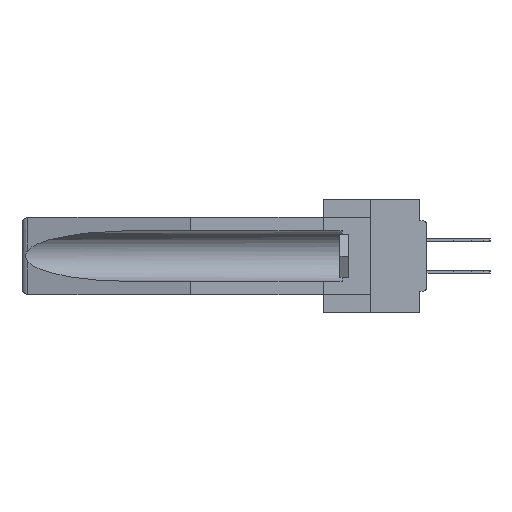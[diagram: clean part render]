
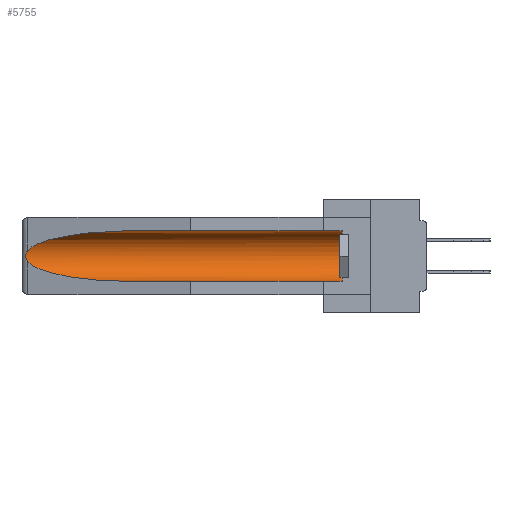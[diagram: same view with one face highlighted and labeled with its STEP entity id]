
A CAD part, left-side view. The second image highlights one B-rep face of the part: STEP entity #5755.
In plain terms, the highlighted cylindrical face has radius 2.857 mm (diameter 5.715 mm), a partial arc.
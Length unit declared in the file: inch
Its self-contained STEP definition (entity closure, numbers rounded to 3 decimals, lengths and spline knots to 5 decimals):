
#371 = CARTESIAN_POINT ( 'NONE',  ( 0.26654, 1.53092, -0.15636 ) ) ;
#1544 = CARTESIAN_POINT ( 'NONE',  ( 0.26537, 1.52718, -0.19328 ) ) ;
#1752 = VERTEX_POINT ( 'NONE', #14575 ) ;
#1980 = CARTESIAN_POINT ( 'NONE',  ( 0.155, 1.07973, -0.284 ) ) ;
#2885 = CARTESIAN_POINT ( 'NONE',  ( 0.155, 1.07973, -0.284 ) ) ;
#3195 = VECTOR ( 'NONE', #3414, 39.37008 ) ;
#3279 = CARTESIAN_POINT ( 'NONE',  ( 0.26597, 1.5296, -0.19026 ) ) ;
#3414 = DIRECTION ( 'NONE',  ( 0., 1., 0. ) ) ;
#3974 = CIRCLE ( 'NONE', #24772, 0.1125 ) ;
#5003 = EDGE_CURVE ( 'NONE', #15911, #29726, #14883, .T. ) ;
#5018 = LINE ( 'NONE', #29493, #3195 ) ;
#5310 = ORIENTED_EDGE ( 'NONE', *, *, #18681, .T. ) ;
#5755 = ADVANCED_FACE ( 'NONE', ( #21621 ), #22930, .F. ) ;
#6008 = EDGE_CURVE ( 'NONE', #31244, #1752, #3974, .T. ) ;
#6218 = CARTESIAN_POINT ( 'NONE',  ( 0.26537, 1.52718, -0.19328 ) ) ;
#6844 = CARTESIAN_POINT ( 'NONE',  ( 0.26537, 1.52718, -0.14972 ) ) ;
#6896 = ORIENTED_EDGE ( 'NONE', *, *, #30049, .F. ) ;
#9110 = CARTESIAN_POINT ( 'NONE',  ( 0.155, 1.07973, -0.059 ) ) ;
#11602 = CARTESIAN_POINT ( 'NONE',  ( 0.26655, 1.53094, -0.18657 ) ) ;
#13022 = ORIENTED_EDGE ( 'NONE', *, *, #6008, .T. ) ;
#13031 = EDGE_CURVE ( 'NONE', #29726, #21503, #30066, .T. ) ;
#13230 = CARTESIAN_POINT ( 'NONE',  ( 0.21114, 1.30732, -0.059 ) ) ;
#13241 =( BOUNDED_CURVE ( )  B_SPLINE_CURVE ( 3, ( #22427, #13230, #33378, #16157 ),
 .UNSPECIFIED., .F., .F. ) 
 B_SPLINE_CURVE_WITH_KNOTS ( ( 4, 4 ),
 ( 4.71239, 6.08839 ),
 .UNSPECIFIED. ) 
 CURVE ( )  GEOMETRIC_REPRESENTATION_ITEM ( )  RATIONAL_B_SPLINE_CURVE ( ( 1., 0.848, 0.848, 1. ) ) 
 REPRESENTATION_ITEM ( '' )  );
#14575 = CARTESIAN_POINT ( 'NONE',  ( 0.155, 0.126, -0.059 ) ) ;
#14738 = DIRECTION ( 'NONE',  ( 0., 1., 0. ) ) ;
#14883 = B_SPLINE_CURVE_WITH_KNOTS ( 'NONE', 3,
 ( #28872, #26458, #371, #23339, #17307, #23476, #29259, #11602, #3279, #6218 ),
 .UNSPECIFIED., .F., .F.,
 ( 4, 2, 2, 2, 4 ),
 ( 0., 0.00029, 0.00058, 0.00087, 0.00117 ),
 .UNSPECIFIED. ) ;
#15911 = VERTEX_POINT ( 'NONE', #6844 ) ;
#16157 = CARTESIAN_POINT ( 'NONE',  ( 0.26537, 1.52718, -0.14972 ) ) ;
#17038 = ORIENTED_EDGE ( 'NONE', *, *, #13031, .T. ) ;
#17307 = CARTESIAN_POINT ( 'NONE',  ( 0.2675, 1.53308, -0.16763 ) ) ;
#18681 = EDGE_CURVE ( 'NONE', #31863, #15911, #13241, .T. ) ;
#20160 = VECTOR ( 'NONE', #24122, 39.37008 ) ;
#20790 = ORIENTED_EDGE ( 'NONE', *, *, #37305, .T. ) ;
#21503 = VERTEX_POINT ( 'NONE', #2885 ) ;
#21621 = FACE_OUTER_BOUND ( 'NONE', #26945, .T. ) ;
#22427 = CARTESIAN_POINT ( 'NONE',  ( 0.155, 1.07973, -0.059 ) ) ;
#22930 = CYLINDRICAL_SURFACE ( 'NONE', #28860, 0.1125 ) ;
#23339 = CARTESIAN_POINT ( 'NONE',  ( 0.2673, 1.5327, -0.16383 ) ) ;
#23476 = CARTESIAN_POINT ( 'NONE',  ( 0.2675, 1.53308, -0.17534 ) ) ;
#24122 = DIRECTION ( 'NONE',  ( 0., 1., 0. ) ) ;
#24772 = AXIS2_PLACEMENT_3D ( 'NONE', #28141, #27768, #25217 ) ;
#25217 = DIRECTION ( 'NONE',  ( 0., 0., 1. ) ) ;
#26458 = CARTESIAN_POINT ( 'NONE',  ( 0.26597, 1.52961, -0.15275 ) ) ;
#26544 = DIRECTION ( 'NONE',  ( 0., 0., 1. ) ) ;
#26945 = EDGE_LOOP ( 'NONE', ( #5310, #31490, #17038, #6896, #13022, #20790 ) ) ;
#27768 = DIRECTION ( 'NONE',  ( 0., -1., 0. ) ) ;
#28141 = CARTESIAN_POINT ( 'NONE',  ( 0.155, 0.126, -0.1715 ) ) ;
#28356 = CARTESIAN_POINT ( 'NONE',  ( 0.25451, 1.48313, -0.24835 ) ) ;
#28860 = AXIS2_PLACEMENT_3D ( 'NONE', #29329, #14738, #26544 ) ;
#28872 = CARTESIAN_POINT ( 'NONE',  ( 0.26537, 1.52718, -0.14972 ) ) ;
#29162 = LINE ( 'NONE', #32328, #20160 ) ;
#29188 = CARTESIAN_POINT ( 'NONE',  ( 0.155, 0.126, -0.284 ) ) ;
#29259 = CARTESIAN_POINT ( 'NONE',  ( 0.2673, 1.53269, -0.17917 ) ) ;
#29329 = CARTESIAN_POINT ( 'NONE',  ( 0.155, -0.30754, -0.1715 ) ) ;
#29493 = CARTESIAN_POINT ( 'NONE',  ( 0.155, -0.30754, -0.284 ) ) ;
#29726 = VERTEX_POINT ( 'NONE', #1544 ) ;
#30049 = EDGE_CURVE ( 'NONE', #31244, #21503, #5018, .T. ) ;
#30066 =( BOUNDED_CURVE ( )  B_SPLINE_CURVE ( 3, ( #33509, #28356, #36795, #1980 ),
 .UNSPECIFIED., .F., .F. ) 
 B_SPLINE_CURVE_WITH_KNOTS ( ( 4, 4 ),
 ( 0.1948, 1.5708 ),
 .UNSPECIFIED. ) 
 CURVE ( )  GEOMETRIC_REPRESENTATION_ITEM ( )  RATIONAL_B_SPLINE_CURVE ( ( 1., 0.848, 0.848, 1. ) ) 
 REPRESENTATION_ITEM ( '' )  );
#31244 = VERTEX_POINT ( 'NONE', #29188 ) ;
#31490 = ORIENTED_EDGE ( 'NONE', *, *, #5003, .T. ) ;
#31863 = VERTEX_POINT ( 'NONE', #9110 ) ;
#32328 = CARTESIAN_POINT ( 'NONE',  ( 0.155, -0.30754, -0.059 ) ) ;
#33378 = CARTESIAN_POINT ( 'NONE',  ( 0.25451, 1.48313, -0.09465 ) ) ;
#33509 = CARTESIAN_POINT ( 'NONE',  ( 0.26537, 1.52718, -0.19328 ) ) ;
#36795 = CARTESIAN_POINT ( 'NONE',  ( 0.21114, 1.30732, -0.284 ) ) ;
#37305 = EDGE_CURVE ( 'NONE', #1752, #31863, #29162, .T. ) ;
